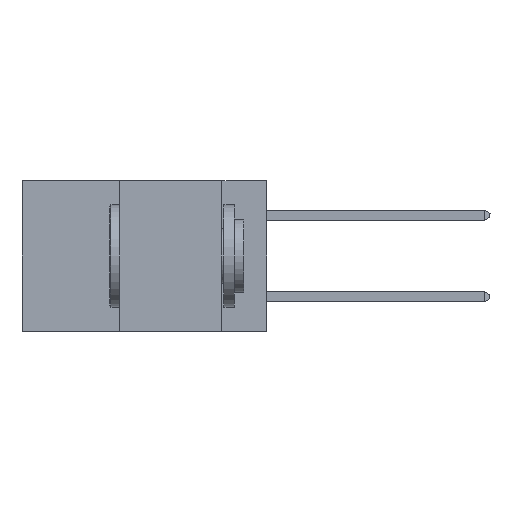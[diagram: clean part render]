
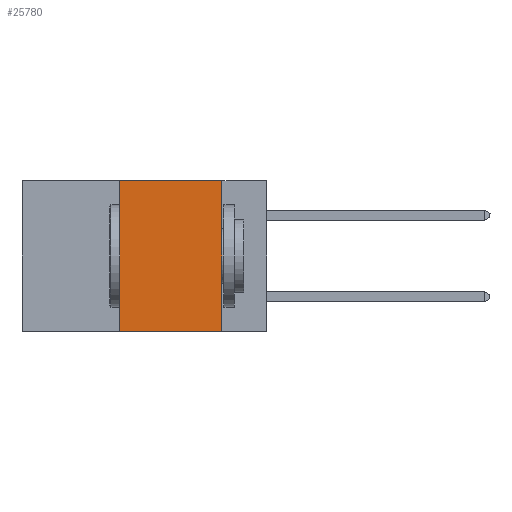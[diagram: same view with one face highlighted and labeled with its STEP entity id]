
A CAD part, left-side view. The second image highlights one B-rep face of the part: STEP entity #25780.
In plain terms, the highlighted planar face has unit normal (-1, 0, 0).
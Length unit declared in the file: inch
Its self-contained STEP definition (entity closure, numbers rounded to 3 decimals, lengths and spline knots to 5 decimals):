
#4699 = CARTESIAN_POINT ( 'NONE',  ( 0., 0.6, 0. ) ) ;
#6005 = LINE ( 'NONE', #21263, #31392 ) ;
#6880 = VECTOR ( 'NONE', #26028, 39.37008 ) ;
#8017 = DIRECTION ( 'NONE',  ( 0., -1., 0. ) ) ;
#8693 = ORIENTED_EDGE ( 'NONE', *, *, #38512, .F. ) ;
#8871 = PLANE ( 'NONE',  #31706 ) ;
#9461 = CARTESIAN_POINT ( 'NONE',  ( 0., 0.11, 0. ) ) ;
#11231 = CARTESIAN_POINT ( 'NONE',  ( 0., 0.11, 0. ) ) ;
#11997 = CARTESIAN_POINT ( 'NONE',  ( 0., 0.36, -0.37 ) ) ;
#13117 = FACE_OUTER_BOUND ( 'NONE', #33912, .T. ) ;
#13543 = VECTOR ( 'NONE', #8017, 39.37008 ) ;
#14399 = ORIENTED_EDGE ( 'NONE', *, *, #15642, .F. ) ;
#14707 = EDGE_CURVE ( 'NONE', #27103, #23209, #16473, .T. ) ;
#15562 = DIRECTION ( 'NONE',  ( 0., 0., -1. ) ) ;
#15642 = EDGE_CURVE ( 'NONE', #23209, #25568, #22376, .T. ) ;
#15956 = CARTESIAN_POINT ( 'NONE',  ( 0., 0.11, -0.37 ) ) ;
#16473 = LINE ( 'NONE', #26537, #24274 ) ;
#18537 = ORIENTED_EDGE ( 'NONE', *, *, #14707, .F. ) ;
#21263 = CARTESIAN_POINT ( 'NONE',  ( 0., 0.6, -0.37 ) ) ;
#22376 = LINE ( 'NONE', #4699, #13543 ) ;
#23187 = DIRECTION ( 'NONE',  ( 0., 0., 1. ) ) ;
#23209 = VERTEX_POINT ( 'NONE', #31116 ) ;
#24274 = VECTOR ( 'NONE', #23187, 39.37008 ) ;
#25568 = VERTEX_POINT ( 'NONE', #11231 ) ;
#25780 = ADVANCED_FACE ( 'NONE', ( #13117 ), #8871, .F. ) ;
#26028 = DIRECTION ( 'NONE',  ( 0., 0., -1. ) ) ;
#26537 = CARTESIAN_POINT ( 'NONE',  ( 0., 0.36, 0. ) ) ;
#27103 = VERTEX_POINT ( 'NONE', #11997 ) ;
#30463 = VERTEX_POINT ( 'NONE', #15956 ) ;
#31116 = CARTESIAN_POINT ( 'NONE',  ( 0., 0.36, 0. ) ) ;
#31392 = VECTOR ( 'NONE', #34754, 39.37008 ) ;
#31706 = AXIS2_PLACEMENT_3D ( 'NONE', #32088, #35436, #15562 ) ;
#32088 = CARTESIAN_POINT ( 'NONE',  ( 0., 0.6, 0. ) ) ;
#33912 = EDGE_LOOP ( 'NONE', ( #8693, #14399, #18537, #36642 ) ) ;
#34754 = DIRECTION ( 'NONE',  ( 0., -1., 0. ) ) ;
#35436 = DIRECTION ( 'NONE',  ( 1., 0., 0. ) ) ;
#36642 = ORIENTED_EDGE ( 'NONE', *, *, #36771, .T. ) ;
#36771 = EDGE_CURVE ( 'NONE', #27103, #30463, #6005, .T. ) ;
#38512 = EDGE_CURVE ( 'NONE', #25568, #30463, #42106, .T. ) ;
#42106 = LINE ( 'NONE', #9461, #6880 ) ;
